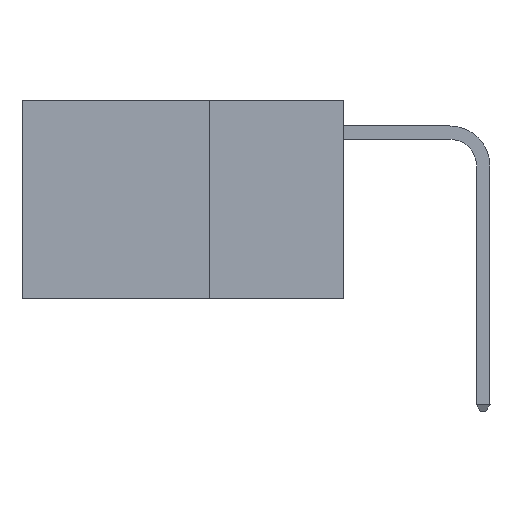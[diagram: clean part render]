
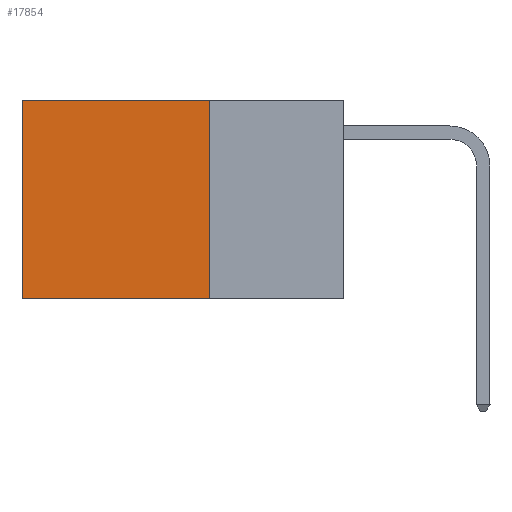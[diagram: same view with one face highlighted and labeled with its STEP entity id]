
A CAD part, left-side view. The second image highlights one B-rep face of the part: STEP entity #17854.
In plain terms, the highlighted planar face has unit normal (-1, 0, 0).
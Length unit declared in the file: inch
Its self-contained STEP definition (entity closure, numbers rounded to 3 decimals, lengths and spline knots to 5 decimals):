
#148 = ORIENTED_EDGE ( 'NONE', *, *, #9079, .F. ) ;
#412 = DIRECTION ( 'NONE',  ( 0., 1., 0. ) ) ;
#442 = CARTESIAN_POINT ( 'NONE',  ( 0.2625, 0.25, 0. ) ) ;
#788 = CARTESIAN_POINT ( 'NONE',  ( 0.2625, 0.25, 0. ) ) ;
#1083 = CARTESIAN_POINT ( 'NONE',  ( 0.2625, 0.6, -0.37 ) ) ;
#1836 = VECTOR ( 'NONE', #12910, 39.37008 ) ;
#2597 = LINE ( 'NONE', #17435, #23595 ) ;
#3135 = ORIENTED_EDGE ( 'NONE', *, *, #18958, .T. ) ;
#3602 = ORIENTED_EDGE ( 'NONE', *, *, #10994, .F. ) ;
#4039 = CARTESIAN_POINT ( 'NONE',  ( 0.2625, 0.25, -0.37 ) ) ;
#4884 = CARTESIAN_POINT ( 'NONE',  ( 0.2625, 0.25, 0. ) ) ;
#5115 = EDGE_CURVE ( 'NONE', #22989, #8803, #2597, .T. ) ;
#8735 = DIRECTION ( 'NONE',  ( 1., 0., 0. ) ) ;
#8803 = VERTEX_POINT ( 'NONE', #1083 ) ;
#9079 = EDGE_CURVE ( 'NONE', #11371, #8803, #20658, .T. ) ;
#10994 = EDGE_CURVE ( 'NONE', #14008, #11371, #21732, .T. ) ;
#11338 = VECTOR ( 'NONE', #412, 39.37008 ) ;
#11371 = VERTEX_POINT ( 'NONE', #23978 ) ;
#11781 = EDGE_LOOP ( 'NONE', ( #22719, #148, #3602, #3135 ) ) ;
#12051 = DIRECTION ( 'NONE',  ( 0., 0., -1. ) ) ;
#12225 = AXIS2_PLACEMENT_3D ( 'NONE', #442, #8735, #15550 ) ;
#12910 = DIRECTION ( 'NONE',  ( 0., 1., 0. ) ) ;
#13371 = FACE_OUTER_BOUND ( 'NONE', #11781, .T. ) ;
#14008 = VERTEX_POINT ( 'NONE', #23118 ) ;
#15281 = PLANE ( 'NONE',  #12225 ) ;
#15550 = DIRECTION ( 'NONE',  ( 0., 0., -1. ) ) ;
#17435 = CARTESIAN_POINT ( 'NONE',  ( 0.2625, 0.6, 0. ) ) ;
#17854 = ADVANCED_FACE ( 'NONE', ( #13371 ), #15281, .F. ) ;
#18958 = EDGE_CURVE ( 'NONE', #14008, #22989, #19058, .T. ) ;
#19058 = LINE ( 'NONE', #4884, #11338 ) ;
#20658 = LINE ( 'NONE', #4039, #1836 ) ;
#21387 = VECTOR ( 'NONE', #12051, 39.37008 ) ;
#21732 = LINE ( 'NONE', #788, #21387 ) ;
#22669 = CARTESIAN_POINT ( 'NONE',  ( 0.2625, 0.6, 0. ) ) ;
#22719 = ORIENTED_EDGE ( 'NONE', *, *, #5115, .T. ) ;
#22989 = VERTEX_POINT ( 'NONE', #22669 ) ;
#23118 = CARTESIAN_POINT ( 'NONE',  ( 0.2625, 0.25, 0. ) ) ;
#23595 = VECTOR ( 'NONE', #25713, 39.37008 ) ;
#23978 = CARTESIAN_POINT ( 'NONE',  ( 0.2625, 0.25, -0.37 ) ) ;
#25713 = DIRECTION ( 'NONE',  ( 0., 0., -1. ) ) ;
